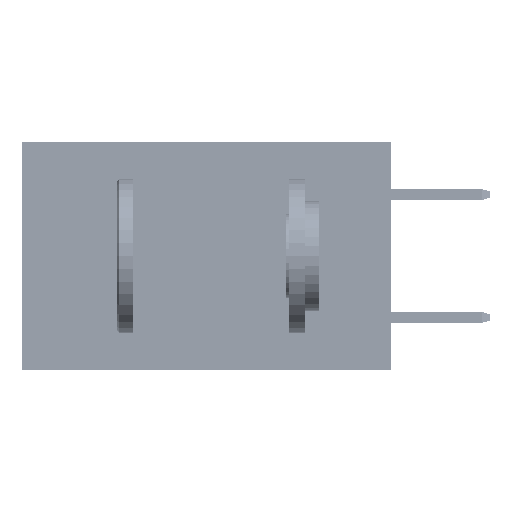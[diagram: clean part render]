
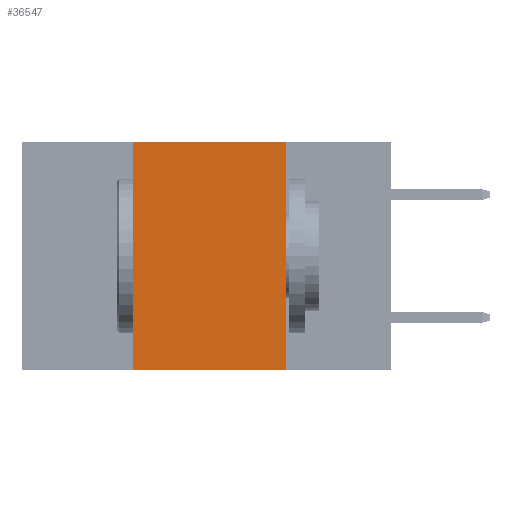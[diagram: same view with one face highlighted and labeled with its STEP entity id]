
A CAD part, left-side view. The second image highlights one B-rep face of the part: STEP entity #36547.
In plain terms, the highlighted planar face has unit normal (-1, 0, 0).
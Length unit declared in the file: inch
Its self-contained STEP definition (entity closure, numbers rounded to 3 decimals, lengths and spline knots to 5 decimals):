
#3598 = ORIENTED_EDGE ( 'NONE', *, *, #33098, .F. ) ;
#5347 = CARTESIAN_POINT ( 'NONE',  ( 0., 0.17, 0. ) ) ;
#6933 = ORIENTED_EDGE ( 'NONE', *, *, #45064, .F. ) ;
#8890 = AXIS2_PLACEMENT_3D ( 'NONE', #11785, #39565, #15775 ) ;
#9203 = LINE ( 'NONE', #49025, #22897 ) ;
#11303 = CARTESIAN_POINT ( 'NONE',  ( 0., 0.42, -0.37 ) ) ;
#11785 = CARTESIAN_POINT ( 'NONE',  ( 0., 0.6, 0. ) ) ;
#13778 = DIRECTION ( 'NONE',  ( 0., 0., -1. ) ) ;
#14628 = EDGE_LOOP ( 'NONE', ( #3598, #6933, #17423, #46560 ) ) ;
#15387 = FACE_OUTER_BOUND ( 'NONE', #14628, .T. ) ;
#15775 = DIRECTION ( 'NONE',  ( 0., 0., -1. ) ) ;
#16151 = DIRECTION ( 'NONE',  ( 0., 0., 1. ) ) ;
#17211 = LINE ( 'NONE', #25129, #50735 ) ;
#17423 = ORIENTED_EDGE ( 'NONE', *, *, #26335, .F. ) ;
#20975 = LINE ( 'NONE', #32820, #28450 ) ;
#21140 = DIRECTION ( 'NONE',  ( 0., -1., 0. ) ) ;
#21299 = LINE ( 'NONE', #36815, #44300 ) ;
#22897 = VECTOR ( 'NONE', #13778, 39.37008 ) ;
#23425 = CARTESIAN_POINT ( 'NONE',  ( 0., 0.17, -0.37 ) ) ;
#25129 = CARTESIAN_POINT ( 'NONE',  ( 0., 0.6, -0.37 ) ) ;
#26335 = EDGE_CURVE ( 'NONE', #50962, #39083, #20975, .T. ) ;
#28418 = EDGE_CURVE ( 'NONE', #50962, #40512, #17211, .T. ) ;
#28450 = VECTOR ( 'NONE', #16151, 39.37008 ) ;
#30105 = CARTESIAN_POINT ( 'NONE',  ( 0., 0.42, 0. ) ) ;
#31268 = PLANE ( 'NONE',  #8890 ) ;
#32820 = CARTESIAN_POINT ( 'NONE',  ( 0., 0.42, 0. ) ) ;
#32988 = DIRECTION ( 'NONE',  ( 0., -1., 0. ) ) ;
#33098 = EDGE_CURVE ( 'NONE', #35452, #40512, #9203, .T. ) ;
#35452 = VERTEX_POINT ( 'NONE', #5347 ) ;
#36547 = ADVANCED_FACE ( 'NONE', ( #15387 ), #31268, .F. ) ;
#36815 = CARTESIAN_POINT ( 'NONE',  ( 0., 0.6, 0. ) ) ;
#39083 = VERTEX_POINT ( 'NONE', #30105 ) ;
#39565 = DIRECTION ( 'NONE',  ( 1., 0., 0. ) ) ;
#40512 = VERTEX_POINT ( 'NONE', #23425 ) ;
#44300 = VECTOR ( 'NONE', #32988, 39.37008 ) ;
#45064 = EDGE_CURVE ( 'NONE', #39083, #35452, #21299, .T. ) ;
#46560 = ORIENTED_EDGE ( 'NONE', *, *, #28418, .T. ) ;
#49025 = CARTESIAN_POINT ( 'NONE',  ( 0., 0.17, 0. ) ) ;
#50735 = VECTOR ( 'NONE', #21140, 39.37008 ) ;
#50962 = VERTEX_POINT ( 'NONE', #11303 ) ;
